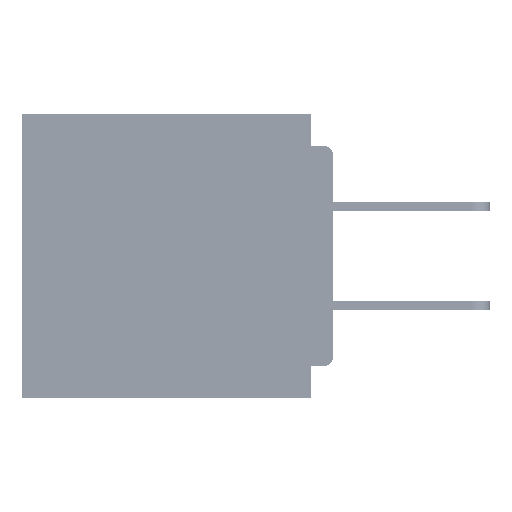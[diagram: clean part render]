
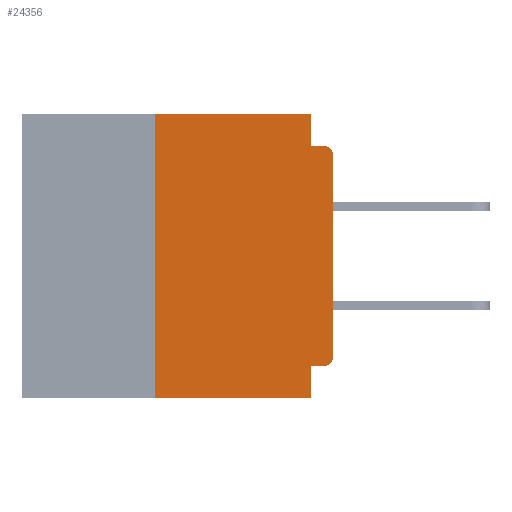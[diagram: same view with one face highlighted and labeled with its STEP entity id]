
A CAD part, left-side view. The second image highlights one B-rep face of the part: STEP entity #24356.
In plain terms, the highlighted planar face has unit normal (-1, 0, 0).
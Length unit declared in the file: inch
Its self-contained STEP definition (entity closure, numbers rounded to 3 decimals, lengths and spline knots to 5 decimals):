
#80 = DIRECTION ( 'NONE',  ( 0., 0., -1. ) ) ;
#1124 = DIRECTION ( 'NONE',  ( 0., 0., -1. ) ) ;
#2020 = CARTESIAN_POINT ( 'NONE',  ( 0., 0., -0.06 ) ) ;
#2359 = ORIENTED_EDGE ( 'NONE', *, *, #65012, .F. ) ;
#5721 = LINE ( 'NONE', #40226, #47378 ) ;
#6778 = DIRECTION ( 'NONE',  ( 0., -1., 0. ) ) ;
#8980 = LINE ( 'NONE', #66102, #36101 ) ;
#10359 = ORIENTED_EDGE ( 'NONE', *, *, #32036, .F. ) ;
#10757 = VECTOR ( 'NONE', #30620, 39.37008 ) ;
#10998 = CARTESIAN_POINT ( 'NONE',  ( 0., 0.437, 0. ) ) ;
#12239 = EDGE_CURVE ( 'NONE', #53394, #59411, #35151, .T. ) ;
#12901 = LINE ( 'NONE', #21061, #67016 ) ;
#13261 = DIRECTION ( 'NONE',  ( 0., -1., 0. ) ) ;
#13288 = AXIS2_PLACEMENT_3D ( 'NONE', #22971, #60827, #28406 ) ;
#14073 = CARTESIAN_POINT ( 'NONE',  ( 0., 0.25, -0.4 ) ) ;
#14186 = DIRECTION ( 'NONE',  ( -1., 0., 0. ) ) ;
#14685 = LINE ( 'NONE', #21633, #40085 ) ;
#16225 = ORIENTED_EDGE ( 'NONE', *, *, #30377, .F. ) ;
#16428 = CARTESIAN_POINT ( 'NONE',  ( 0., 0.031, -0.4 ) ) ;
#18236 = VERTEX_POINT ( 'NONE', #50343 ) ;
#18442 = EDGE_CURVE ( 'NONE', #19506, #42490, #61678, .T. ) ;
#18633 = VERTEX_POINT ( 'NONE', #16428 ) ;
#19262 = EDGE_CURVE ( 'NONE', #29087, #18236, #66601, .T. ) ;
#19506 = VERTEX_POINT ( 'NONE', #60889 ) ;
#21061 = CARTESIAN_POINT ( 'NONE',  ( 0., 0., -0.355 ) ) ;
#21162 = VERTEX_POINT ( 'NONE', #31306 ) ;
#21633 = CARTESIAN_POINT ( 'NONE',  ( 0., 0., 0. ) ) ;
#22971 = CARTESIAN_POINT ( 'NONE',  ( 0., 0.015, -0.06 ) ) ;
#23485 = ORIENTED_EDGE ( 'NONE', *, *, #18442, .F. ) ;
#24030 = CARTESIAN_POINT ( 'NONE',  ( 0., 0.031, 0. ) ) ;
#24356 = ADVANCED_FACE ( 'NONE', ( #48561 ), #48904, .F. ) ;
#24582 = ORIENTED_EDGE ( 'NONE', *, *, #12239, .T. ) ;
#24904 = EDGE_CURVE ( 'NONE', #61588, #50884, #12901, .T. ) ;
#25180 = CARTESIAN_POINT ( 'NONE',  ( 0., 0.031, 0. ) ) ;
#27688 = LINE ( 'NONE', #29927, #40436 ) ;
#28381 = CARTESIAN_POINT ( 'NONE',  ( 0., 0.437, -0.4 ) ) ;
#28406 = DIRECTION ( 'NONE',  ( 0., 0., -1. ) ) ;
#29087 = VERTEX_POINT ( 'NONE', #24030 ) ;
#29927 = CARTESIAN_POINT ( 'NONE',  ( 0., 0.437, 0. ) ) ;
#30035 = ORIENTED_EDGE ( 'NONE', *, *, #19262, .F. ) ;
#30377 = EDGE_CURVE ( 'NONE', #18236, #59411, #5721, .T. ) ;
#30620 = DIRECTION ( 'NONE',  ( 0., 0., -1. ) ) ;
#31306 = CARTESIAN_POINT ( 'NONE',  ( 0., 0., -0.34 ) ) ;
#32036 = EDGE_CURVE ( 'NONE', #42490, #29087, #27688, .T. ) ;
#32718 = DIRECTION ( 'NONE',  ( 1., 0., 0. ) ) ;
#34486 = EDGE_CURVE ( 'NONE', #19506, #18633, #63307, .T. ) ;
#34700 = EDGE_CURVE ( 'NONE', #61588, #21162, #64118, .T. ) ;
#35151 = CIRCLE ( 'NONE', #13288, 0.015 ) ;
#35878 = CARTESIAN_POINT ( 'NONE',  ( 0., 0.015, -0.355 ) ) ;
#36068 = ORIENTED_EDGE ( 'NONE', *, *, #58278, .T. ) ;
#36101 = VECTOR ( 'NONE', #1124, 39.37008 ) ;
#40085 = VECTOR ( 'NONE', #70330, 39.37008 ) ;
#40226 = CARTESIAN_POINT ( 'NONE',  ( 0., 0., -0.045 ) ) ;
#40379 = ORIENTED_EDGE ( 'NONE', *, *, #34700, .T. ) ;
#40436 = VECTOR ( 'NONE', #40839, 39.37008 ) ;
#40839 = DIRECTION ( 'NONE',  ( 0., -1., 0. ) ) ;
#42490 = VERTEX_POINT ( 'NONE', #59055 ) ;
#45146 = CARTESIAN_POINT ( 'NONE',  ( 0., 0.031, -0.355 ) ) ;
#46630 = CARTESIAN_POINT ( 'NONE',  ( 0., 0.015, -0.34 ) ) ;
#47352 = VECTOR ( 'NONE', #51960, 39.37008 ) ;
#47378 = VECTOR ( 'NONE', #13261, 39.37008 ) ;
#48561 = FACE_OUTER_BOUND ( 'NONE', #63463, .T. ) ;
#48904 = PLANE ( 'NONE',  #55814 ) ;
#48985 = VECTOR ( 'NONE', #6778, 39.37008 ) ;
#50343 = CARTESIAN_POINT ( 'NONE',  ( 0., 0.031, -0.045 ) ) ;
#50884 = VERTEX_POINT ( 'NONE', #45146 ) ;
#51960 = DIRECTION ( 'NONE',  ( 0., 0., 1. ) ) ;
#52074 = DIRECTION ( 'NONE',  ( 0., 0., -1. ) ) ;
#52091 = ORIENTED_EDGE ( 'NONE', *, *, #34486, .T. ) ;
#52433 = ORIENTED_EDGE ( 'NONE', *, *, #24904, .F. ) ;
#53394 = VERTEX_POINT ( 'NONE', #2020 ) ;
#55814 = AXIS2_PLACEMENT_3D ( 'NONE', #10998, #32718, #80 ) ;
#58278 = EDGE_CURVE ( 'NONE', #21162, #53394, #14685, .T. ) ;
#59055 = CARTESIAN_POINT ( 'NONE',  ( 0., 0.25, 0. ) ) ;
#59411 = VERTEX_POINT ( 'NONE', #60562 ) ;
#60562 = CARTESIAN_POINT ( 'NONE',  ( 0., 0.015, -0.045 ) ) ;
#60827 = DIRECTION ( 'NONE',  ( -1., 0., 0. ) ) ;
#60889 = CARTESIAN_POINT ( 'NONE',  ( 0., 0.25, -0.4 ) ) ;
#61588 = VERTEX_POINT ( 'NONE', #35878 ) ;
#61678 = LINE ( 'NONE', #14073, #47352 ) ;
#62992 = AXIS2_PLACEMENT_3D ( 'NONE', #46630, #14186, #52074 ) ;
#63307 = LINE ( 'NONE', #28381, #48985 ) ;
#63463 = EDGE_LOOP ( 'NONE', ( #36068, #24582, #16225, #30035, #10359, #23485, #52091, #2359, #52433, #40379 ) ) ;
#64118 = CIRCLE ( 'NONE', #62992, 0.015 ) ;
#64338 = DIRECTION ( 'NONE',  ( 0., 1., 0. ) ) ;
#65012 = EDGE_CURVE ( 'NONE', #50884, #18633, #8980, .T. ) ;
#66102 = CARTESIAN_POINT ( 'NONE',  ( 0., 0.031, -0.4 ) ) ;
#66601 = LINE ( 'NONE', #25180, #10757 ) ;
#67016 = VECTOR ( 'NONE', #64338, 39.37008 ) ;
#70330 = DIRECTION ( 'NONE',  ( 0., 0., 1. ) ) ;
